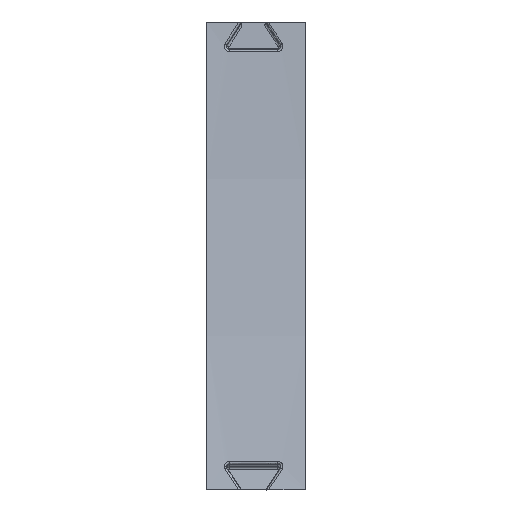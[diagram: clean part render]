
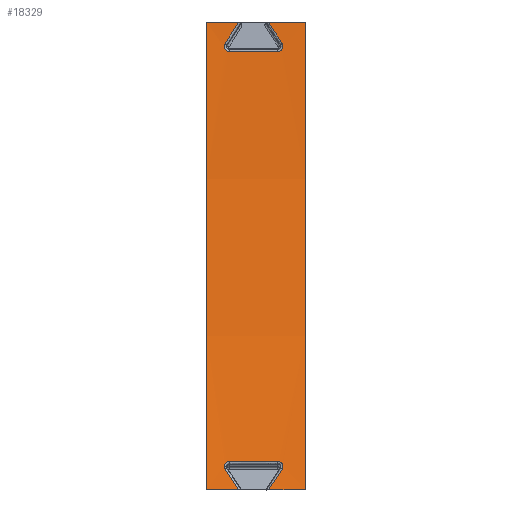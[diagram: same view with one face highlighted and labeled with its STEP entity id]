
A CAD part, left-side view. The second image highlights one B-rep face of the part: STEP entity #18329.
In plain terms, the highlighted cylindrical face has radius 949 mm (diameter 1898 mm), a partial arc.
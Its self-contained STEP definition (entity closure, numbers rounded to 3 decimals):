
#67=ELLIPSE('',#18982,1119.255,949.);
#68=ELLIPSE('',#18986,1119.289,949.);
#70=ELLIPSE('',#18990,1119.289,949.);
#71=ELLIPSE('',#18991,1119.289,949.);
#120=CYLINDRICAL_SURFACE('',#18989,949.);
#201=CIRCLE('',#18953,949.);
#214=CIRCLE('',#18992,949.);
#1223=B_SPLINE_CURVE_WITH_KNOTS('',3,(#33759,#33760,#33761,#33762,#33763,
#33764,#33765),.UNSPECIFIED.,.F.,.F.,(4,1,1,1,4),(-0.373,-0.293,
-0.213,-0.106,0.),
 .UNSPECIFIED.);
#1225=B_SPLINE_CURVE_WITH_KNOTS('',3,(#33796,#33797,#33798,#33799),
 .UNSPECIFIED.,.F.,.F.,(4,4),(-0.82,0.82),
 .UNSPECIFIED.);
#1227=B_SPLINE_CURVE_WITH_KNOTS('',3,(#33842,#33843,#33844,#33845,#33846,
#33847,#33848),.UNSPECIFIED.,.F.,.F.,(4,1,1,1,4),(-0.373,-0.266,
-0.16,-0.08,0.),
 .UNSPECIFIED.);
#1232=B_SPLINE_CURVE_WITH_KNOTS('',3,(#33912,#33913,#33914,#33915),
 .UNSPECIFIED.,.F.,.F.,(4,4),(-2.307,-2.199),
 .UNSPECIFIED.);
#1233=B_SPLINE_CURVE_WITH_KNOTS('',3,(#33917,#33918,#33919,#33920,#33921),
 .UNSPECIFIED.,.F.,.F.,(4,1,4),(-1.1,-0.987,-0.836),
 .UNSPECIFIED.);
#1234=B_SPLINE_CURVE_WITH_KNOTS('',3,(#33923,#33924,#33925,#33926),
 .UNSPECIFIED.,.F.,.F.,(4,4),(-0.82,0.82),
 .UNSPECIFIED.);
#1235=B_SPLINE_CURVE_WITH_KNOTS('',3,(#33928,#33929,#33930,#33931,#33932,
#33933,#33934),.UNSPECIFIED.,.F.,.F.,(4,1,1,1,4),(-0.373,-0.266,
-0.16,-0.08,0.),
 .UNSPECIFIED.);
#2513=FACE_OUTER_BOUND('',#3597,.T.);
#3597=EDGE_LOOP('',(#16030,#16031,#16032,#16033,#16034,#16035,#16036,#16037,
#16038,#16039,#16040,#16041,#16042,#16043,#16044,#16045,#16046));
#5238=LINE('',#33906,#6885);
#5239=LINE('',#33908,#6886);
#5240=LINE('',#33938,#6887);
#5241=LINE('',#33941,#6888);
#6885=VECTOR('',#21703,10.);
#6886=VECTOR('',#21704,10.);
#6887=VECTOR('',#21709,10.);
#6888=VECTOR('',#21712,10.);
#8555=VERTEX_POINT('',#33585);
#8557=VERTEX_POINT('',#33589);
#8576=VERTEX_POINT('',#33707);
#8577=VERTEX_POINT('',#33709);
#8579=VERTEX_POINT('',#33757);
#8581=VERTEX_POINT('',#33794);
#8583=VERTEX_POINT('',#33840);
#8585=VERTEX_POINT('',#33877);
#8588=VERTEX_POINT('',#33907);
#8589=VERTEX_POINT('',#33909);
#8590=VERTEX_POINT('',#33911);
#8591=VERTEX_POINT('',#33916);
#8592=VERTEX_POINT('',#33922);
#8593=VERTEX_POINT('',#33927);
#8594=VERTEX_POINT('',#33935);
#8595=VERTEX_POINT('',#33937);
#8596=VERTEX_POINT('',#33939);
#11072=EDGE_CURVE('',#8555,#8557,#201,.T.);
#11096=EDGE_CURVE('',#8576,#8577,#67,.T.);
#11099=EDGE_CURVE('',#8579,#8576,#1223,.T.);
#11102=EDGE_CURVE('',#8581,#8579,#1225,.T.);
#11105=EDGE_CURVE('',#8583,#8581,#1227,.T.);
#11108=EDGE_CURVE('',#8585,#8583,#68,.T.);
#11114=EDGE_CURVE('',#8555,#8585,#5238,.T.);
#11115=EDGE_CURVE('',#8557,#8588,#5239,.T.);
#11116=EDGE_CURVE('',#8589,#8588,#70,.T.);
#11117=EDGE_CURVE('',#8590,#8589,#1232,.T.);
#11118=EDGE_CURVE('',#8591,#8590,#1233,.T.);
#11119=EDGE_CURVE('',#8592,#8591,#1234,.T.);
#11120=EDGE_CURVE('',#8593,#8592,#1235,.T.);
#11121=EDGE_CURVE('',#8594,#8593,#71,.T.);
#11122=EDGE_CURVE('',#8594,#8595,#5240,.T.);
#11123=EDGE_CURVE('',#8596,#8595,#214,.T.);
#11124=EDGE_CURVE('',#8577,#8596,#5241,.T.);
#16030=ORIENTED_EDGE('',*,*,#11096,.F.);
#16031=ORIENTED_EDGE('',*,*,#11099,.F.);
#16032=ORIENTED_EDGE('',*,*,#11102,.F.);
#16033=ORIENTED_EDGE('',*,*,#11105,.F.);
#16034=ORIENTED_EDGE('',*,*,#11108,.F.);
#16035=ORIENTED_EDGE('',*,*,#11114,.F.);
#16036=ORIENTED_EDGE('',*,*,#11072,.T.);
#16037=ORIENTED_EDGE('',*,*,#11115,.T.);
#16038=ORIENTED_EDGE('',*,*,#11116,.F.);
#16039=ORIENTED_EDGE('',*,*,#11117,.F.);
#16040=ORIENTED_EDGE('',*,*,#11118,.F.);
#16041=ORIENTED_EDGE('',*,*,#11119,.F.);
#16042=ORIENTED_EDGE('',*,*,#11120,.F.);
#16043=ORIENTED_EDGE('',*,*,#11121,.F.);
#16044=ORIENTED_EDGE('',*,*,#11122,.T.);
#16045=ORIENTED_EDGE('',*,*,#11123,.F.);
#16046=ORIENTED_EDGE('',*,*,#11124,.F.);
#18329=ADVANCED_FACE('',(#2513),#120,.F.);
#18953=AXIS2_PLACEMENT_3D('',#33591,#21617,#21618);
#18982=AXIS2_PLACEMENT_3D('',#33710,#21685,#21686);
#18986=AXIS2_PLACEMENT_3D('',#33890,#21693,#21694);
#18989=AXIS2_PLACEMENT_3D('',#33905,#21701,#21702);
#18990=AXIS2_PLACEMENT_3D('',#33910,#21705,#21706);
#18991=AXIS2_PLACEMENT_3D('',#33936,#21707,#21708);
#18992=AXIS2_PLACEMENT_3D('',#33940,#21710,#21711);
#21617=DIRECTION('center_axis',(0.,1.,0.));
#21618=DIRECTION('ref_axis',(1.,0.,-0.031));
#21685=DIRECTION('center_axis',(0.046,-0.848,0.528));
#21686=DIRECTION('ref_axis',(-0.074,-0.53,-0.845));
#21693=DIRECTION('center_axis',(0.046,0.848,0.528));
#21694=DIRECTION('ref_axis',(-0.074,0.53,-0.845));
#21701=DIRECTION('center_axis',(0.,1.,0.));
#21702=DIRECTION('ref_axis',(1.,0.,-0.031));
#21703=DIRECTION('',(0.,-1.,0.));
#21704=DIRECTION('',(0.,-1.,0.));
#21705=DIRECTION('center_axis',(-0.137,0.848,-0.512));
#21706=DIRECTION('ref_axis',(0.219,0.53,0.819));
#21707=DIRECTION('center_axis',(-0.137,-0.848,-0.512));
#21708=DIRECTION('ref_axis',(0.219,-0.53,0.819));
#21709=DIRECTION('',(0.,-1.,0.));
#21710=DIRECTION('center_axis',(0.,1.,0.));
#21711=DIRECTION('ref_axis',(1.,0.,-0.031));
#21712=DIRECTION('',(0.,-1.,0.));
#33585=CARTESIAN_POINT('',(-103.794,39.734,-81.334));
#33589=CARTESIAN_POINT('',(-131.781,39.734,-240.077));
#33591=CARTESIAN_POINT('Origin',(-1048.998,39.734,3.472));
#33707=CARTESIAN_POINT('',(-104.48,14.069,-88.663));
#33709=CARTESIAN_POINT('',(-103.794,18.671,-81.334));
#33710=CARTESIAN_POINT('Origin',(-1048.998,19.987,3.472));
#33757=CARTESIAN_POINT('',(-104.744,15.552,-91.325));
#33759=CARTESIAN_POINT('Ctrl Pts',(-104.744,15.552,-91.325));
#33760=CARTESIAN_POINT('Ctrl Pts',(-104.744,15.286,-91.325));
#33761=CARTESIAN_POINT('Ctrl Pts',(-104.731,14.755,-91.202));
#33762=CARTESIAN_POINT('Ctrl Pts',(-104.674,14.048,-90.63));
#33763=CARTESIAN_POINT('Ctrl Pts',(-104.58,13.694,-89.677));
#33764=CARTESIAN_POINT('Ctrl Pts',(-104.509,13.881,-88.962));
#33765=CARTESIAN_POINT('Ctrl Pts',(-104.48,14.069,-88.663));
#33794=CARTESIAN_POINT('',(-104.745,31.944,-91.333));
#33796=CARTESIAN_POINT('Ctrl Pts',(-104.745,31.944,-91.333));
#33797=CARTESIAN_POINT('Ctrl Pts',(-104.744,26.48,-91.33));
#33798=CARTESIAN_POINT('Ctrl Pts',(-104.744,21.016,-91.328));
#33799=CARTESIAN_POINT('Ctrl Pts',(-104.744,15.552,-91.325));
#33840=CARTESIAN_POINT('',(-104.481,33.429,-88.67));
#33842=CARTESIAN_POINT('Ctrl Pts',(-104.481,33.429,-88.67));
#33843=CARTESIAN_POINT('Ctrl Pts',(-104.51,33.617,-88.97));
#33844=CARTESIAN_POINT('Ctrl Pts',(-104.58,33.804,-89.686));
#33845=CARTESIAN_POINT('Ctrl Pts',(-104.675,33.449,-90.638));
#33846=CARTESIAN_POINT('Ctrl Pts',(-104.732,32.742,-91.21));
#33847=CARTESIAN_POINT('Ctrl Pts',(-104.745,32.21,-91.333));
#33848=CARTESIAN_POINT('Ctrl Pts',(-104.745,31.944,-91.333));
#33877=CARTESIAN_POINT('',(-103.794,28.821,-81.334));
#33890=CARTESIAN_POINT('Origin',(-1048.998,27.505,3.472));
#33905=CARTESIAN_POINT('Origin',(-1048.998,22.926,3.472));
#33906=CARTESIAN_POINT('',(-103.794,22.926,-81.334));
#33907=CARTESIAN_POINT('',(-131.781,28.85,-240.077));
#33908=CARTESIAN_POINT('',(-131.781,22.926,-240.077));
#33909=CARTESIAN_POINT('',(-129.929,33.429,-232.992));
#33910=CARTESIAN_POINT('Origin',(-1048.998,27.51,3.472));
#33911=CARTESIAN_POINT('',(-129.673,33.692,-231.994));
#33912=CARTESIAN_POINT('Ctrl Pts',(-129.673,33.692,-231.994));
#33913=CARTESIAN_POINT('Ctrl Pts',(-129.762,33.713,-232.342));
#33914=CARTESIAN_POINT('Ctrl Pts',(-129.853,33.62,-232.696));
#33915=CARTESIAN_POINT('Ctrl Pts',(-129.929,33.429,-232.992));
#33916=CARTESIAN_POINT('',(-129.269,31.947,-230.409));
#33917=CARTESIAN_POINT('Ctrl Pts',(-129.269,31.947,-230.409));
#33918=CARTESIAN_POINT('Ctrl Pts',(-129.269,32.323,-230.409));
#33919=CARTESIAN_POINT('Ctrl Pts',(-129.341,33.202,-230.693));
#33920=CARTESIAN_POINT('Ctrl Pts',(-129.549,33.66,-231.509));
#33921=CARTESIAN_POINT('Ctrl Pts',(-129.673,33.692,-231.994));
#33922=CARTESIAN_POINT('',(-129.267,15.555,-230.401));
#33923=CARTESIAN_POINT('Ctrl Pts',(-129.267,15.555,-230.401));
#33924=CARTESIAN_POINT('Ctrl Pts',(-129.267,21.019,-230.403));
#33925=CARTESIAN_POINT('Ctrl Pts',(-129.268,26.483,-230.406));
#33926=CARTESIAN_POINT('Ctrl Pts',(-129.269,31.947,-230.409));
#33927=CARTESIAN_POINT('',(-129.93,14.07,-232.993));
#33928=CARTESIAN_POINT('Ctrl Pts',(-129.93,14.07,-232.993));
#33929=CARTESIAN_POINT('Ctrl Pts',(-129.855,13.882,-232.701));
#33930=CARTESIAN_POINT('Ctrl Pts',(-129.676,13.695,-232.005));
#33931=CARTESIAN_POINT('Ctrl Pts',(-129.439,14.05,-231.077));
#33932=CARTESIAN_POINT('Ctrl Pts',(-129.297,14.757,-230.52));
#33933=CARTESIAN_POINT('Ctrl Pts',(-129.267,15.289,-230.401));
#33934=CARTESIAN_POINT('Ctrl Pts',(-129.267,15.555,-230.401));
#33935=CARTESIAN_POINT('',(-131.781,18.649,-240.077));
#33936=CARTESIAN_POINT('Origin',(-1048.998,19.989,3.472));
#33937=CARTESIAN_POINT('',(-131.781,6.118,-240.077));
#33938=CARTESIAN_POINT('',(-131.781,22.926,-240.077));
#33939=CARTESIAN_POINT('',(-103.794,6.118,-81.334));
#33940=CARTESIAN_POINT('Origin',(-1048.998,6.118,3.472));
#33941=CARTESIAN_POINT('',(-103.794,22.926,-81.334));
